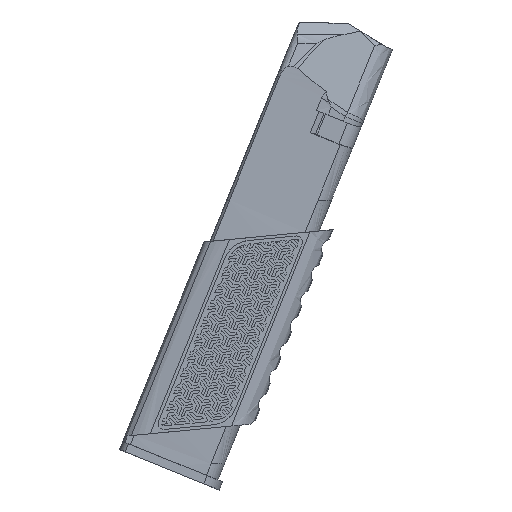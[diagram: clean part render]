
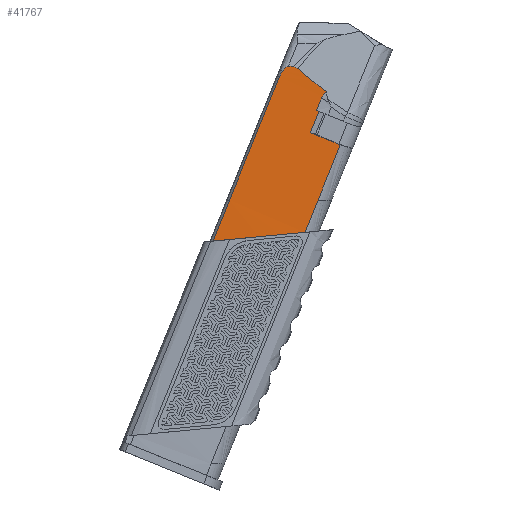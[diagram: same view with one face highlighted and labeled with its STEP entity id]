
A CAD part, front view. The second image highlights one B-rep face of the part: STEP entity #41767.
In plain terms, the highlighted cylindrical face has radius 941.89 mm (diameter 1883.78 mm), a partial arc.
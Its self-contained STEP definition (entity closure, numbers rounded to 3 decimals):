
#103=CYLINDRICAL_SURFACE('',#44016,941.89);
#221=ELLIPSE('',#44017,1061.869,941.89);
#222=ELLIPSE('',#44018,945.656,941.89);
#223=ELLIPSE('',#44019,945.656,941.89);
#224=ELLIPSE('',#44020,3587.87,941.89);
#225=ELLIPSE('',#44021,7108.15,941.89);
#226=ELLIPSE('',#44022,5554.111,941.89);
#4643=FACE_OUTER_BOUND('',#6924,.T.);
#6924=EDGE_LOOP('',(#36997,#36998,#36999,#37000,#37001,#37002,#37003,#37004,
#37005,#37006,#37007,#37008,#37009,#37010,#37011));
#11062=LINE('',#93775,#15065);
#11063=LINE('',#93869,#15066);
#11066=LINE('',#93904,#15069);
#11067=LINE('',#93908,#15070);
#11068=LINE('',#93912,#15071);
#11069=LINE('',#93945,#15072);
#15065=VECTOR('',#52113,10.);
#15066=VECTOR('',#52116,10.);
#15069=VECTOR('',#52127,10.);
#15070=VECTOR('',#52130,10.);
#15071=VECTOR('',#52133,10.);
#15072=VECTOR('',#52140,10.);
#17158=B_SPLINE_CURVE_WITH_KNOTS('',3,(#93918,#93919,#93920,#93921,#93922,
#93923),.UNSPECIFIED.,.F.,.F.,(4,2,4),(0.586,0.614,
0.707),.UNSPECIFIED.);
#17159=B_SPLINE_CURVE_WITH_KNOTS('',3,(#93927,#93928,#93929,#93930,#93931,
#93932,#93933,#93934,#93935,#93936),.UNSPECIFIED.,.F.,.F.,(4,2,2,2,4),(-0.263,
-0.24,-0.212,-0.131,0.),
 .UNSPECIFIED.);
#17160=B_SPLINE_CURVE_WITH_KNOTS('',3,(#93938,#93939,#93940,#93941,#93942,
#93943,#93944),.UNSPECIFIED.,.F.,.F.,(4,3,4),(-0.22,-0.108,
0.),.UNSPECIFIED.);
#21008=VERTEX_POINT('',#93763);
#21009=VERTEX_POINT('',#93774);
#21010=VERTEX_POINT('',#93787);
#21011=VERTEX_POINT('',#93798);
#21015=VERTEX_POINT('',#93903);
#21016=VERTEX_POINT('',#93905);
#21017=VERTEX_POINT('',#93907);
#21018=VERTEX_POINT('',#93909);
#21019=VERTEX_POINT('',#93911);
#21020=VERTEX_POINT('',#93913);
#21021=VERTEX_POINT('',#93915);
#21022=VERTEX_POINT('',#93917);
#21023=VERTEX_POINT('',#93924);
#21024=VERTEX_POINT('',#93926);
#21025=VERTEX_POINT('',#93937);
#26944=EDGE_CURVE('',#21008,#21009,#11062,.T.);
#26948=EDGE_CURVE('',#21011,#21010,#11063,.T.);
#26954=EDGE_CURVE('',#21010,#21008,#221,.F.);
#26955=EDGE_CURVE('',#21015,#21011,#11066,.T.);
#26956=EDGE_CURVE('',#21016,#21015,#222,.F.);
#26957=EDGE_CURVE('',#21017,#21016,#11067,.T.);
#26958=EDGE_CURVE('',#21017,#21018,#223,.F.);
#26959=EDGE_CURVE('',#21018,#21019,#11068,.T.);
#26960=EDGE_CURVE('',#21019,#21020,#224,.T.);
#26961=EDGE_CURVE('',#21020,#21021,#225,.T.);
#26962=EDGE_CURVE('',#21021,#21022,#17158,.T.);
#26963=EDGE_CURVE('',#21022,#21023,#226,.T.);
#26964=EDGE_CURVE('',#21023,#21024,#17159,.T.);
#26965=EDGE_CURVE('',#21024,#21025,#17160,.T.);
#26966=EDGE_CURVE('',#21009,#21025,#11069,.T.);
#36997=ORIENTED_EDGE('',*,*,#26954,.F.);
#36998=ORIENTED_EDGE('',*,*,#26948,.F.);
#36999=ORIENTED_EDGE('',*,*,#26955,.F.);
#37000=ORIENTED_EDGE('',*,*,#26956,.F.);
#37001=ORIENTED_EDGE('',*,*,#26957,.F.);
#37002=ORIENTED_EDGE('',*,*,#26958,.T.);
#37003=ORIENTED_EDGE('',*,*,#26959,.T.);
#37004=ORIENTED_EDGE('',*,*,#26960,.T.);
#37005=ORIENTED_EDGE('',*,*,#26961,.T.);
#37006=ORIENTED_EDGE('',*,*,#26962,.T.);
#37007=ORIENTED_EDGE('',*,*,#26963,.T.);
#37008=ORIENTED_EDGE('',*,*,#26964,.T.);
#37009=ORIENTED_EDGE('',*,*,#26965,.T.);
#37010=ORIENTED_EDGE('',*,*,#26966,.F.);
#37011=ORIENTED_EDGE('',*,*,#26944,.F.);
#41767=ADVANCED_FACE('',(#4643),#103,.T.);
#44016=AXIS2_PLACEMENT_3D('',#93901,#52123,#52124);
#44017=AXIS2_PLACEMENT_3D('',#93902,#52125,#52126);
#44018=AXIS2_PLACEMENT_3D('',#93906,#52128,#52129);
#44019=AXIS2_PLACEMENT_3D('',#93910,#52131,#52132);
#44020=AXIS2_PLACEMENT_3D('',#93914,#52134,#52135);
#44021=AXIS2_PLACEMENT_3D('',#93916,#52136,#52137);
#44022=AXIS2_PLACEMENT_3D('',#93925,#52138,#52139);
#52113=DIRECTION('',(0.376,0.,0.927));
#52116=DIRECTION('',(-0.376,0.,-0.927));
#52123=DIRECTION('center_axis',(-0.376,0.,
-0.927));
#52124=DIRECTION('ref_axis',(0.031,0.999,-0.013));
#52125=DIRECTION('center_axis',(-0.095,0.,
0.996));
#52126=DIRECTION('ref_axis',(0.996,0.,0.095));
#52127=DIRECTION('',(-0.376,0.,-0.927));
#52128=DIRECTION('center_axis',(-0.374,0.089,-0.923));
#52129=DIRECTION('ref_axis',(0.035,0.996,0.082));
#52130=DIRECTION('',(-0.378,0.,-0.926));
#52131=DIRECTION('center_axis',(0.374,-0.089,0.923));
#52132=DIRECTION('ref_axis',(0.035,0.996,0.082));
#52133=DIRECTION('',(0.376,0.,0.927));
#52134=DIRECTION('center_axis',(-0.668,-0.497,0.554));
#52135=DIRECTION('ref_axis',(0.571,0.135,0.81));
#52136=DIRECTION('center_axis',(-0.075,0.991,-0.113));
#52137=DIRECTION('ref_axis',(0.369,0.132,0.92));
#52138=DIRECTION('center_axis',(0.,0.983,-0.183));
#52139=DIRECTION('ref_axis',(0.381,0.169,0.909));
#52140=DIRECTION('',(0.376,0.,0.927));
#93763=CARTESIAN_POINT('',(77.406,11.819,90.414));
#93774=CARTESIAN_POINT('',(83.103,11.819,104.462));
#93775=CARTESIAN_POINT('',(36.511,11.819,-10.433));
#93787=CARTESIAN_POINT('',(108.887,11.553,93.404));
#93798=CARTESIAN_POINT('',(113.371,11.553,104.462));
#93869=CARTESIAN_POINT('',(62.504,11.553,-20.974));
#93901=CARTESIAN_POINT('Origin',(57.799,953.429,-19.065));
#93902=CARTESIAN_POINT('Origin',(103.188,953.429,92.863));
#93903=CARTESIAN_POINT('',(121.018,11.553,123.321));
#93904=CARTESIAN_POINT('',(93.199,11.553,54.718));
#93905=CARTESIAN_POINT('',(110.727,11.559,127.493));
#93906=CARTESIAN_POINT('Origin',(147.998,953.429,203.365));
#93907=CARTESIAN_POINT('',(113.698,11.559,134.775));
#93908=CARTESIAN_POINT('',(113.698,11.559,134.775));
#93909=CARTESIAN_POINT('',(112.813,11.565,135.134));
#93910=CARTESIAN_POINT('Origin',(150.954,953.429,210.653));
#93911=CARTESIAN_POINT('',(114.531,11.565,139.37));
#93912=CARTESIAN_POINT('',(82.038,11.565,59.244));
#93913=CARTESIAN_POINT('',(116.291,11.559,141.487));
#93914=CARTESIAN_POINT('Origin',(799.429,953.429,1809.782));
#93915=CARTESIAN_POINT('',(106.263,11.72,149.594));
#93916=CARTESIAN_POINT('Origin',(2768.09,953.429,6664.465));
#93917=CARTESIAN_POINT('',(105.136,11.745,150.044));
#93918=CARTESIAN_POINT('Ctrl Pts',(106.263,11.72,149.594));
#93919=CARTESIAN_POINT('Ctrl Pts',(106.192,11.722,149.656));
#93920=CARTESIAN_POINT('Ctrl Pts',(106.117,11.724,149.711));
#93921=CARTESIAN_POINT('Ctrl Pts',(105.774,11.732,149.921));
#93922=CARTESIAN_POINT('Ctrl Pts',(105.462,11.738,150.009));
#93923=CARTESIAN_POINT('Ctrl Pts',(105.136,11.745,150.044));
#93924=CARTESIAN_POINT('',(103.234,11.785,150.261));
#93925=CARTESIAN_POINT('Origin',(2177.887,953.429,5209.035));
#93926=CARTESIAN_POINT('',(101.233,11.814,148.527));
#93927=CARTESIAN_POINT('Ctrl Pts',(103.234,11.785,150.261));
#93928=CARTESIAN_POINT('Ctrl Pts',(103.159,11.787,150.27));
#93929=CARTESIAN_POINT('Ctrl Pts',(103.083,11.789,150.259));
#93930=CARTESIAN_POINT('Ctrl Pts',(102.919,11.792,150.213));
#93931=CARTESIAN_POINT('Ctrl Pts',(102.828,11.793,150.169));
#93932=CARTESIAN_POINT('Ctrl Pts',(102.515,11.798,149.983));
#93933=CARTESIAN_POINT('Ctrl Pts',(102.283,11.802,149.769));
#93934=CARTESIAN_POINT('Ctrl Pts',(101.792,11.808,149.262));
#93935=CARTESIAN_POINT('Ctrl Pts',(101.492,11.811,148.881));
#93936=CARTESIAN_POINT('Ctrl Pts',(101.233,11.814,148.527));
#93937=CARTESIAN_POINT('',(100.183,11.819,146.581));
#93938=CARTESIAN_POINT('Ctrl Pts',(101.233,11.814,148.527));
#93939=CARTESIAN_POINT('Ctrl Pts',(101.014,11.816,148.227));
#93940=CARTESIAN_POINT('Ctrl Pts',(100.816,11.817,147.898));
#93941=CARTESIAN_POINT('Ctrl Pts',(100.642,11.818,147.57));
#93942=CARTESIAN_POINT('Ctrl Pts',(100.473,11.819,147.251));
#93943=CARTESIAN_POINT('Ctrl Pts',(100.319,11.819,146.916));
#93944=CARTESIAN_POINT('Ctrl Pts',(100.183,11.819,146.581));
#93945=CARTESIAN_POINT('',(67.206,11.819,65.259));
